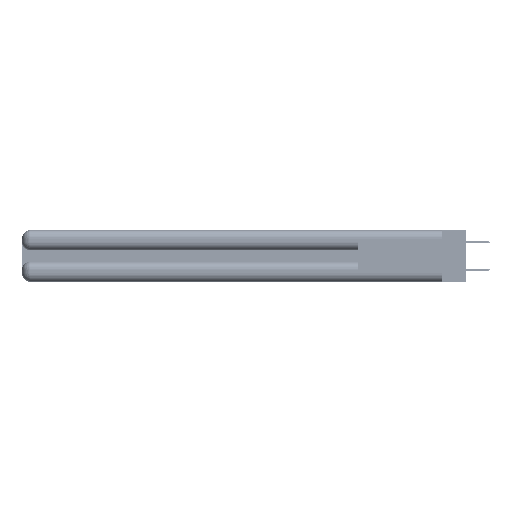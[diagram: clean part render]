
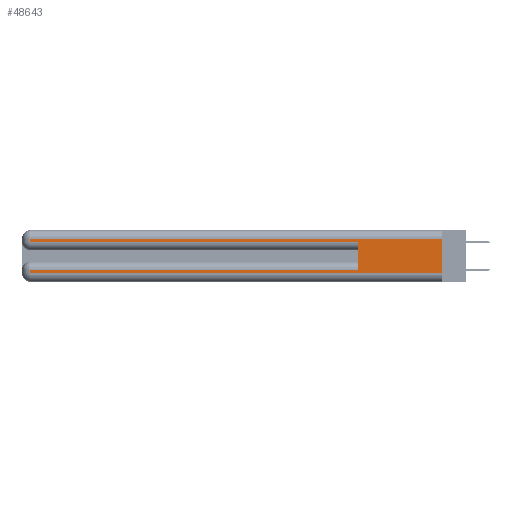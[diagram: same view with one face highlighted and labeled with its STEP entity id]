
A CAD part, left-side view. The second image highlights one B-rep face of the part: STEP entity #48643.
In plain terms, the highlighted planar face has unit normal (-1, 0, 0).
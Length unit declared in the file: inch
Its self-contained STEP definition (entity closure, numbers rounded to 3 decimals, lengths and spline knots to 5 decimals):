
#939 = CARTESIAN_POINT ( 'NONE',  ( 0., 0., 0.37 ) ) ;
#1280 = ORIENTED_EDGE ( 'NONE', *, *, #17773, .F. ) ;
#1343 = PLANE ( 'NONE',  #6942 ) ;
#1840 = VECTOR ( 'NONE', #37541, 39.37008 ) ;
#3593 = LINE ( 'NONE', #939, #35023 ) ;
#5825 = DIRECTION ( 'NONE',  ( 1., 0., 0. ) ) ;
#6942 = AXIS2_PLACEMENT_3D ( 'NONE', #45954, #5825, #37070 ) ;
#8892 = DIRECTION ( 'NONE',  ( 0., 0., -1. ) ) ;
#8994 = CARTESIAN_POINT ( 'NONE',  ( 0., 0., 0.285 ) ) ;
#10612 = VERTEX_POINT ( 'NONE', #23022 ) ;
#11100 = CARTESIAN_POINT ( 'NONE',  ( 0., 0., 0.31 ) ) ;
#13693 = LINE ( 'NONE', #23996, #1840 ) ;
#13772 = VERTEX_POINT ( 'NONE', #24938 ) ;
#16165 = FACE_OUTER_BOUND ( 'NONE', #31433, .T. ) ;
#16883 = VERTEX_POINT ( 'NONE', #45956 ) ;
#17332 = ORIENTED_EDGE ( 'NONE', *, *, #51682, .T. ) ;
#17570 = LINE ( 'NONE', #55276, #39989 ) ;
#17773 = EDGE_CURVE ( 'NONE', #47089, #13772, #28115, .T. ) ;
#17998 = ORIENTED_EDGE ( 'NONE', *, *, #38581, .T. ) ;
#18725 = ORIENTED_EDGE ( 'NONE', *, *, #34685, .T. ) ;
#23022 = CARTESIAN_POINT ( 'NONE',  ( 0., 2.94, 0.06 ) ) ;
#23548 = VECTOR ( 'NONE', #51566, 39.37008 ) ;
#23607 = ORIENTED_EDGE ( 'NONE', *, *, #45043, .T. ) ;
#23996 = CARTESIAN_POINT ( 'NONE',  ( 0., 0., 0.085 ) ) ;
#24938 = CARTESIAN_POINT ( 'NONE',  ( 0., 0.6, 0.285 ) ) ;
#25669 = ORIENTED_EDGE ( 'NONE', *, *, #27624, .F. ) ;
#26486 = CARTESIAN_POINT ( 'NONE',  ( 0., 0., 0.31 ) ) ;
#26693 = VECTOR ( 'NONE', #52695, 39.37008 ) ;
#26738 = LINE ( 'NONE', #26486, #49257 ) ;
#27624 = EDGE_CURVE ( 'NONE', #37035, #48548, #3593, .T. ) ;
#27939 = CARTESIAN_POINT ( 'NONE',  ( 0., 2.94, 0.285 ) ) ;
#28115 = LINE ( 'NONE', #39348, #26693 ) ;
#29473 = LINE ( 'NONE', #40134, #51962 ) ;
#29875 = ORIENTED_EDGE ( 'NONE', *, *, #40112, .T. ) ;
#30208 = VECTOR ( 'NONE', #40218, 39.37008 ) ;
#30942 = CARTESIAN_POINT ( 'NONE',  ( 0., 0.6, 0.085 ) ) ;
#30981 = DIRECTION ( 'NONE',  ( 0., 1., 0. ) ) ;
#31433 = EDGE_LOOP ( 'NONE', ( #25669, #17998, #29875, #23607, #1280, #17332, #18725, #46834 ) ) ;
#31771 = CARTESIAN_POINT ( 'NONE',  ( 0., 0., 0.06 ) ) ;
#32945 = DIRECTION ( 'NONE',  ( 0., -1., 0. ) ) ;
#34685 = EDGE_CURVE ( 'NONE', #40832, #10612, #35468, .T. ) ;
#35023 = VECTOR ( 'NONE', #36696, 39.37008 ) ;
#35468 = LINE ( 'NONE', #38016, #23548 ) ;
#35764 = CARTESIAN_POINT ( 'NONE',  ( 0., 2.94, 0.085 ) ) ;
#36696 = DIRECTION ( 'NONE',  ( 0., 0., -1. ) ) ;
#37035 = VERTEX_POINT ( 'NONE', #11100 ) ;
#37070 = DIRECTION ( 'NONE',  ( 0., 0., -1. ) ) ;
#37541 = DIRECTION ( 'NONE',  ( 0., 1., 0. ) ) ;
#38016 = CARTESIAN_POINT ( 'NONE',  ( 0., 2.94, 0.37 ) ) ;
#38581 = EDGE_CURVE ( 'NONE', #37035, #16883, #26738, .T. ) ;
#39348 = CARTESIAN_POINT ( 'NONE',  ( 0., 0.6, 0.145 ) ) ;
#39989 = VECTOR ( 'NONE', #32945, 39.37008 ) ;
#40112 = EDGE_CURVE ( 'NONE', #16883, #49624, #29473, .T. ) ;
#40134 = CARTESIAN_POINT ( 'NONE',  ( 0., 2.94, 0.37 ) ) ;
#40218 = DIRECTION ( 'NONE',  ( 0., -1., 0. ) ) ;
#40832 = VERTEX_POINT ( 'NONE', #35764 ) ;
#45043 = EDGE_CURVE ( 'NONE', #49624, #13772, #51290, .T. ) ;
#45954 = CARTESIAN_POINT ( 'NONE',  ( 0., 0., 0.37 ) ) ;
#45956 = CARTESIAN_POINT ( 'NONE',  ( 0., 2.94, 0.31 ) ) ;
#46834 = ORIENTED_EDGE ( 'NONE', *, *, #56740, .T. ) ;
#47089 = VERTEX_POINT ( 'NONE', #30942 ) ;
#48548 = VERTEX_POINT ( 'NONE', #31771 ) ;
#48643 = ADVANCED_FACE ( 'NONE', ( #16165 ), #1343, .F. ) ;
#49257 = VECTOR ( 'NONE', #30981, 39.37008 ) ;
#49624 = VERTEX_POINT ( 'NONE', #27939 ) ;
#51290 = LINE ( 'NONE', #8994, #30208 ) ;
#51566 = DIRECTION ( 'NONE',  ( 0., 0., -1. ) ) ;
#51682 = EDGE_CURVE ( 'NONE', #47089, #40832, #13693, .T. ) ;
#51962 = VECTOR ( 'NONE', #8892, 39.37008 ) ;
#52695 = DIRECTION ( 'NONE',  ( 0., 0., 1. ) ) ;
#55276 = CARTESIAN_POINT ( 'NONE',  ( 0., 0., 0.06 ) ) ;
#56740 = EDGE_CURVE ( 'NONE', #10612, #48548, #17570, .T. ) ;
